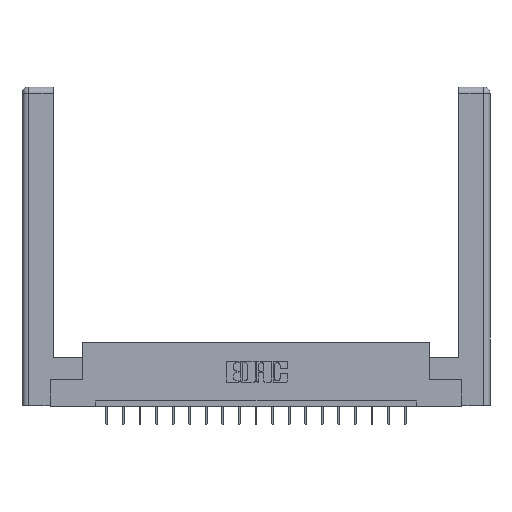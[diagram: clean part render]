
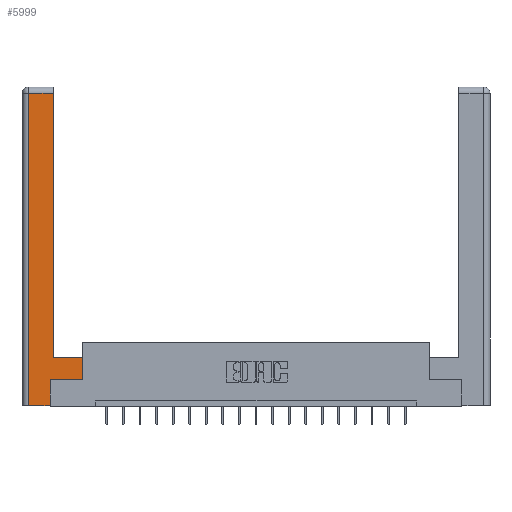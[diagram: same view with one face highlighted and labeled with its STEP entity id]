
A CAD part, top view. The second image highlights one B-rep face of the part: STEP entity #5999.
In plain terms, the highlighted planar face has unit normal (0, 0, 1).
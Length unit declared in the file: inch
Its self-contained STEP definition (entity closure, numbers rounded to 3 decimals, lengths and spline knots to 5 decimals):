
#18 = CARTESIAN_POINT ( 'NONE',  ( 0.565, 0.45, 0. ) ) ;
#612 = DIRECTION ( 'NONE',  ( 1., 0., 0. ) ) ;
#775 = VERTEX_POINT ( 'NONE', #5333 ) ;
#812 = CARTESIAN_POINT ( 'NONE',  ( 0.265, 0., 0. ) ) ;
#875 = EDGE_LOOP ( 'NONE', ( #15450, #13946, #8854, #16339, #16822, #10271, #2442, #19251 ) ) ;
#1279 = VERTEX_POINT ( 'NONE', #13992 ) ;
#1789 = LINE ( 'NONE', #812, #7064 ) ;
#2006 = CARTESIAN_POINT ( 'NONE',  ( 0.565, 0.245, 0. ) ) ;
#2442 = ORIENTED_EDGE ( 'NONE', *, *, #11853, .T. ) ;
#2791 = FACE_OUTER_BOUND ( 'NONE', #875, .T. ) ;
#3071 = LINE ( 'NONE', #15990, #5964 ) ;
#3196 = PLANE ( 'NONE',  #16000 ) ;
#3263 = DIRECTION ( 'NONE',  ( -1., 0., 0. ) ) ;
#3728 = DIRECTION ( 'NONE',  ( 0., 1., 0. ) ) ;
#3764 = VERTEX_POINT ( 'NONE', #18959 ) ;
#3937 = EDGE_CURVE ( 'NONE', #10959, #8841, #13232, .T. ) ;
#4402 = LINE ( 'NONE', #9329, #12526 ) ;
#4748 = CARTESIAN_POINT ( 'NONE',  ( 0., 0., 0. ) ) ;
#5156 = VECTOR ( 'NONE', #15993, 39.37008 ) ;
#5333 = CARTESIAN_POINT ( 'NONE',  ( 0.265, 0., 0. ) ) ;
#5818 = LINE ( 'NONE', #10724, #6989 ) ;
#5964 = VECTOR ( 'NONE', #3728, 39.37008 ) ;
#5999 = ADVANCED_FACE ( 'NONE', ( #2791 ), #3196, .F. ) ;
#6028 = VECTOR ( 'NONE', #7490, 39.37008 ) ;
#6418 = CARTESIAN_POINT ( 'NONE',  ( 0.0615, 0., 0. ) ) ;
#6524 = EDGE_CURVE ( 'NONE', #1279, #10262, #16902, .T. ) ;
#6989 = VECTOR ( 'NONE', #9386, 39.37008 ) ;
#7064 = VECTOR ( 'NONE', #612, 39.37008 ) ;
#7268 = VECTOR ( 'NONE', #10812, 39.37008 ) ;
#7490 = DIRECTION ( 'NONE',  ( -1., 0., 0. ) ) ;
#7592 = EDGE_CURVE ( 'NONE', #3764, #8226, #17064, .T. ) ;
#7601 = EDGE_CURVE ( 'NONE', #8841, #3764, #4402, .T. ) ;
#7752 = CARTESIAN_POINT ( 'NONE',  ( 0.0615, 2.94, 0. ) ) ;
#8226 = VERTEX_POINT ( 'NONE', #11494 ) ;
#8565 = DIRECTION ( 'NONE',  ( 0., -1., 0. ) ) ;
#8841 = VERTEX_POINT ( 'NONE', #16790 ) ;
#8854 = ORIENTED_EDGE ( 'NONE', *, *, #14304, .T. ) ;
#9329 = CARTESIAN_POINT ( 'NONE',  ( 0.295, 3., 0. ) ) ;
#9386 = DIRECTION ( 'NONE',  ( 0., 1., 0. ) ) ;
#9510 = LINE ( 'NONE', #17655, #10495 ) ;
#10262 = VERTEX_POINT ( 'NONE', #2006 ) ;
#10271 = ORIENTED_EDGE ( 'NONE', *, *, #6524, .T. ) ;
#10495 = VECTOR ( 'NONE', #8565, 39.37008 ) ;
#10724 = CARTESIAN_POINT ( 'NONE',  ( 0.565, 0.45, 0. ) ) ;
#10812 = DIRECTION ( 'NONE',  ( -1., 0., 0. ) ) ;
#10959 = VERTEX_POINT ( 'NONE', #18 ) ;
#11494 = CARTESIAN_POINT ( 'NONE',  ( 0.0615, 2.94, 0. ) ) ;
#11853 = EDGE_CURVE ( 'NONE', #10262, #10959, #5818, .T. ) ;
#12526 = VECTOR ( 'NONE', #18502, 39.37008 ) ;
#12704 = CARTESIAN_POINT ( 'NONE',  ( 0.565, 0.245, 0. ) ) ;
#13232 = LINE ( 'NONE', #16660, #6028 ) ;
#13946 = ORIENTED_EDGE ( 'NONE', *, *, #7592, .T. ) ;
#13992 = CARTESIAN_POINT ( 'NONE',  ( 0.265, 0.245, 0. ) ) ;
#14047 = DIRECTION ( 'NONE',  ( 0., 0., -1. ) ) ;
#14304 = EDGE_CURVE ( 'NONE', #8226, #19161, #9510, .T. ) ;
#14454 = EDGE_CURVE ( 'NONE', #775, #1279, #3071, .T. ) ;
#15450 = ORIENTED_EDGE ( 'NONE', *, *, #7601, .T. ) ;
#15990 = CARTESIAN_POINT ( 'NONE',  ( 0.265, 0.245, 0. ) ) ;
#15993 = DIRECTION ( 'NONE',  ( 1., 0., 0. ) ) ;
#16000 = AXIS2_PLACEMENT_3D ( 'NONE', #4748, #14047, #3263 ) ;
#16339 = ORIENTED_EDGE ( 'NONE', *, *, #19329, .T. ) ;
#16660 = CARTESIAN_POINT ( 'NONE',  ( 0.295, 0.45, 0. ) ) ;
#16790 = CARTESIAN_POINT ( 'NONE',  ( 0.295, 0.45, 0. ) ) ;
#16822 = ORIENTED_EDGE ( 'NONE', *, *, #14454, .T. ) ;
#16902 = LINE ( 'NONE', #12704, #5156 ) ;
#17064 = LINE ( 'NONE', #7752, #7268 ) ;
#17655 = CARTESIAN_POINT ( 'NONE',  ( 0.0615, 0., 0. ) ) ;
#18502 = DIRECTION ( 'NONE',  ( 0., 1., 0. ) ) ;
#18959 = CARTESIAN_POINT ( 'NONE',  ( 0.295, 2.94, 0. ) ) ;
#19161 = VERTEX_POINT ( 'NONE', #6418 ) ;
#19251 = ORIENTED_EDGE ( 'NONE', *, *, #3937, .T. ) ;
#19329 = EDGE_CURVE ( 'NONE', #19161, #775, #1789, .T. ) ;
